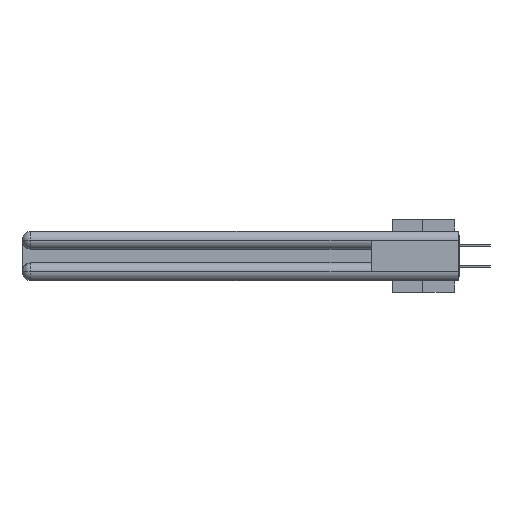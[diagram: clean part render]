
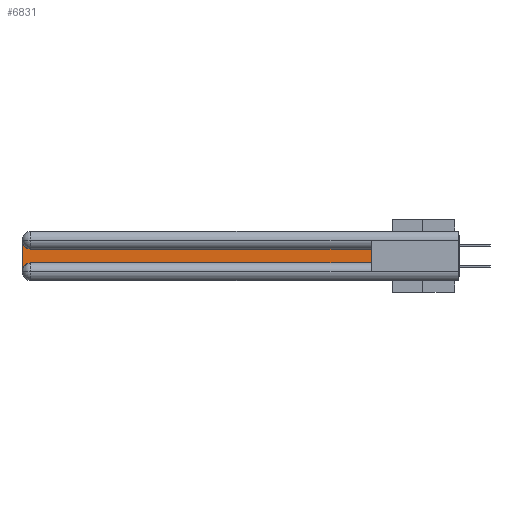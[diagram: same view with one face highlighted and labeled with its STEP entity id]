
A CAD part, left-side view. The second image highlights one B-rep face of the part: STEP entity #6831.
In plain terms, the highlighted planar face has unit normal (-1, 0, 0).
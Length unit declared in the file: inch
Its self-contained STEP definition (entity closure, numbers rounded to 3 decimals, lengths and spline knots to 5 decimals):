
#774 = CARTESIAN_POINT ( 'NONE',  ( 0.075, 0.6, -0.1225 ) ) ;
#1411 = VERTEX_POINT ( 'NONE', #2376 ) ;
#2376 = CARTESIAN_POINT ( 'NONE',  ( 0.075, 2.94, -0.2175 ) ) ;
#2566 = CARTESIAN_POINT ( 'NONE',  ( 0.075, 0.6, -0.2175 ) ) ;
#2985 = EDGE_LOOP ( 'NONE', ( #16743, #45395, #21220, #38444, #43272, #33884 ) ) ;
#3028 = VECTOR ( 'NONE', #26884, 39.37008 ) ;
#3193 = CARTESIAN_POINT ( 'NONE',  ( 0.075, 2.94, -0.2775 ) ) ;
#4902 = CARTESIAN_POINT ( 'NONE',  ( 0.075, 2.94, -0.0625 ) ) ;
#5426 = FACE_OUTER_BOUND ( 'NONE', #2985, .T. ) ;
#6413 = DIRECTION ( 'NONE',  ( 0., 1., 0. ) ) ;
#6831 = ADVANCED_FACE ( 'NONE', ( #5426 ), #28140, .F. ) ;
#6920 = DIRECTION ( 'NONE',  ( 1., 0., 0. ) ) ;
#8978 = VERTEX_POINT ( 'NONE', #2566 ) ;
#9320 = EDGE_CURVE ( 'NONE', #1411, #8978, #27026, .T. ) ;
#11140 = VERTEX_POINT ( 'NONE', #29840 ) ;
#11186 = LINE ( 'NONE', #27055, #3028 ) ;
#11814 = LINE ( 'NONE', #24553, #33755 ) ;
#16369 = AXIS2_PLACEMENT_3D ( 'NONE', #4902, #19319, #42160 ) ;
#16743 = ORIENTED_EDGE ( 'NONE', *, *, #31342, .T. ) ;
#17443 = DIRECTION ( 'NONE',  ( 0., 0., -1. ) ) ;
#18150 = DIRECTION ( 'NONE',  ( 0., 0., -1. ) ) ;
#19319 = DIRECTION ( 'NONE',  ( 1., 0., 0. ) ) ;
#19715 = CIRCLE ( 'NONE', #33278, 0.06 ) ;
#20464 = EDGE_CURVE ( 'NONE', #40444, #11140, #32595, .T. ) ;
#21220 = ORIENTED_EDGE ( 'NONE', *, *, #20464, .T. ) ;
#24524 = EDGE_CURVE ( 'NONE', #11140, #1411, #19715, .T. ) ;
#24553 = CARTESIAN_POINT ( 'NONE',  ( 0.075, 0.6, -0.1225 ) ) ;
#26877 = CIRCLE ( 'NONE', #16369, 0.06 ) ;
#26884 = DIRECTION ( 'NONE',  ( 0., 0., 1. ) ) ;
#27026 = LINE ( 'NONE', #32662, #28245 ) ;
#27055 = CARTESIAN_POINT ( 'NONE',  ( 0.075, 0.6, -0.2175 ) ) ;
#27132 = CARTESIAN_POINT ( 'NONE',  ( 0.075, 2.94, -0.1225 ) ) ;
#28140 = PLANE ( 'NONE',  #45443 ) ;
#28245 = VECTOR ( 'NONE', #44109, 39.37008 ) ;
#29840 = CARTESIAN_POINT ( 'NONE',  ( 0.075, 3., -0.2775 ) ) ;
#30776 = VERTEX_POINT ( 'NONE', #27132 ) ;
#31342 = EDGE_CURVE ( 'NONE', #33237, #30776, #11814, .T. ) ;
#31514 = CARTESIAN_POINT ( 'NONE',  ( 0.075, 3., -0.1225 ) ) ;
#32595 = LINE ( 'NONE', #39468, #39571 ) ;
#32662 = CARTESIAN_POINT ( 'NONE',  ( 0.075, 0.6, -0.2175 ) ) ;
#33237 = VERTEX_POINT ( 'NONE', #774 ) ;
#33278 = AXIS2_PLACEMENT_3D ( 'NONE', #3193, #6920, #18150 ) ;
#33755 = VECTOR ( 'NONE', #6413, 39.37008 ) ;
#33884 = ORIENTED_EDGE ( 'NONE', *, *, #36053, .T. ) ;
#35059 = DIRECTION ( 'NONE',  ( 0., 0., -1. ) ) ;
#35203 = EDGE_CURVE ( 'NONE', #30776, #40444, #26877, .T. ) ;
#36053 = EDGE_CURVE ( 'NONE', #8978, #33237, #11186, .T. ) ;
#38444 = ORIENTED_EDGE ( 'NONE', *, *, #24524, .T. ) ;
#39468 = CARTESIAN_POINT ( 'NONE',  ( 0.075, 3., -0.2175 ) ) ;
#39571 = VECTOR ( 'NONE', #17443, 39.37008 ) ;
#40444 = VERTEX_POINT ( 'NONE', #43448 ) ;
#42160 = DIRECTION ( 'NONE',  ( 0., 0., -1. ) ) ;
#43272 = ORIENTED_EDGE ( 'NONE', *, *, #9320, .T. ) ;
#43448 = CARTESIAN_POINT ( 'NONE',  ( 0.075, 3., -0.0625 ) ) ;
#44109 = DIRECTION ( 'NONE',  ( 0., -1., 0. ) ) ;
#45395 = ORIENTED_EDGE ( 'NONE', *, *, #35203, .T. ) ;
#45443 = AXIS2_PLACEMENT_3D ( 'NONE', #31514, #46054, #35059 ) ;
#46054 = DIRECTION ( 'NONE',  ( 1., 0., 0. ) ) ;
